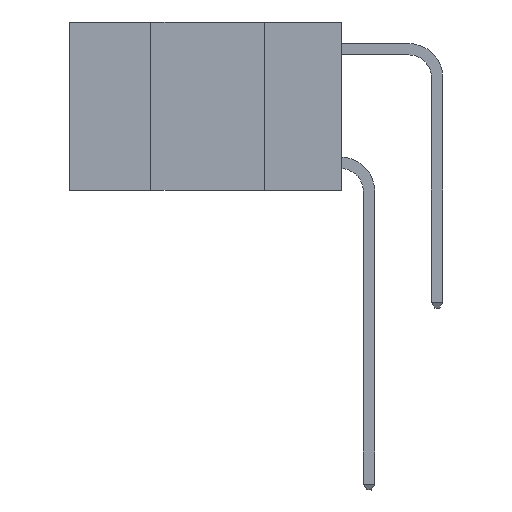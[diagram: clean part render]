
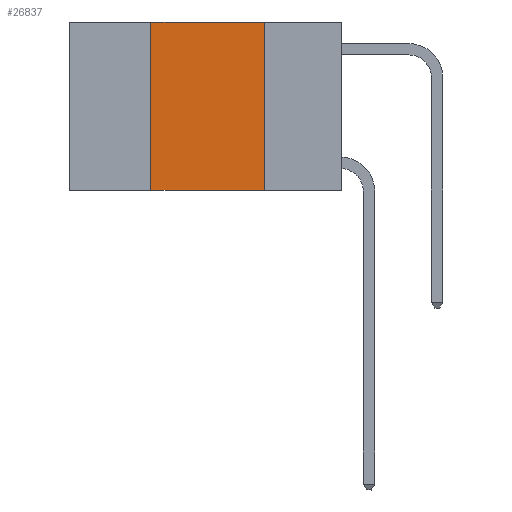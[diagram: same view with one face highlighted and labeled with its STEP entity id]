
A CAD part, left-side view. The second image highlights one B-rep face of the part: STEP entity #26837.
In plain terms, the highlighted planar face has unit normal (-1, 0, 0).
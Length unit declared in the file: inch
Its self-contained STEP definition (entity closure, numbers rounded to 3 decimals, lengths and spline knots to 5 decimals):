
#539 = LINE ( 'NONE', #5169, #17477 ) ;
#850 = VECTOR ( 'NONE', #22817, 39.37008 ) ;
#941 = DIRECTION ( 'NONE',  ( 0., 0., -1. ) ) ;
#1198 = CARTESIAN_POINT ( 'NONE',  ( 0., 0.6, -0.37 ) ) ;
#2390 = CARTESIAN_POINT ( 'NONE',  ( 0., 0.17, 0. ) ) ;
#3242 = CARTESIAN_POINT ( 'NONE',  ( 0., 0.6, 0. ) ) ;
#4264 = VERTEX_POINT ( 'NONE', #27190 ) ;
#5169 = CARTESIAN_POINT ( 'NONE',  ( 0., 0.42, 0. ) ) ;
#7241 = VERTEX_POINT ( 'NONE', #14226 ) ;
#7972 = LINE ( 'NONE', #1198, #19610 ) ;
#7979 = DIRECTION ( 'NONE',  ( 1., 0., 0. ) ) ;
#8876 = ORIENTED_EDGE ( 'NONE', *, *, #17185, .F. ) ;
#8915 = DIRECTION ( 'NONE',  ( 0., 0., -1. ) ) ;
#9077 = EDGE_CURVE ( 'NONE', #10279, #7241, #539, .T. ) ;
#10279 = VERTEX_POINT ( 'NONE', #23235 ) ;
#11386 = VERTEX_POINT ( 'NONE', #24213 ) ;
#11406 = EDGE_LOOP ( 'NONE', ( #8876, #25760, #28723, #28838 ) ) ;
#11879 = LINE ( 'NONE', #2390, #24709 ) ;
#14226 = CARTESIAN_POINT ( 'NONE',  ( 0., 0.42, 0. ) ) ;
#17185 = EDGE_CURVE ( 'NONE', #11386, #4264, #11879, .T. ) ;
#17477 = VECTOR ( 'NONE', #23115, 39.37008 ) ;
#18928 = PLANE ( 'NONE',  #25662 ) ;
#19291 = DIRECTION ( 'NONE',  ( 0., -1., 0. ) ) ;
#19610 = VECTOR ( 'NONE', #19291, 39.37008 ) ;
#21280 = FACE_OUTER_BOUND ( 'NONE', #11406, .T. ) ;
#22817 = DIRECTION ( 'NONE',  ( 0., -1., 0. ) ) ;
#23115 = DIRECTION ( 'NONE',  ( 0., 0., 1. ) ) ;
#23235 = CARTESIAN_POINT ( 'NONE',  ( 0., 0.42, -0.37 ) ) ;
#24097 = EDGE_CURVE ( 'NONE', #7241, #11386, #25340, .T. ) ;
#24213 = CARTESIAN_POINT ( 'NONE',  ( 0., 0.17, 0. ) ) ;
#24218 = EDGE_CURVE ( 'NONE', #10279, #4264, #7972, .T. ) ;
#24709 = VECTOR ( 'NONE', #8915, 39.37008 ) ;
#25340 = LINE ( 'NONE', #27431, #850 ) ;
#25662 = AXIS2_PLACEMENT_3D ( 'NONE', #3242, #7979, #941 ) ;
#25760 = ORIENTED_EDGE ( 'NONE', *, *, #24097, .F. ) ;
#26837 = ADVANCED_FACE ( 'NONE', ( #21280 ), #18928, .F. ) ;
#27190 = CARTESIAN_POINT ( 'NONE',  ( 0., 0.17, -0.37 ) ) ;
#27431 = CARTESIAN_POINT ( 'NONE',  ( 0., 0.6, 0. ) ) ;
#28723 = ORIENTED_EDGE ( 'NONE', *, *, #9077, .F. ) ;
#28838 = ORIENTED_EDGE ( 'NONE', *, *, #24218, .T. ) ;
